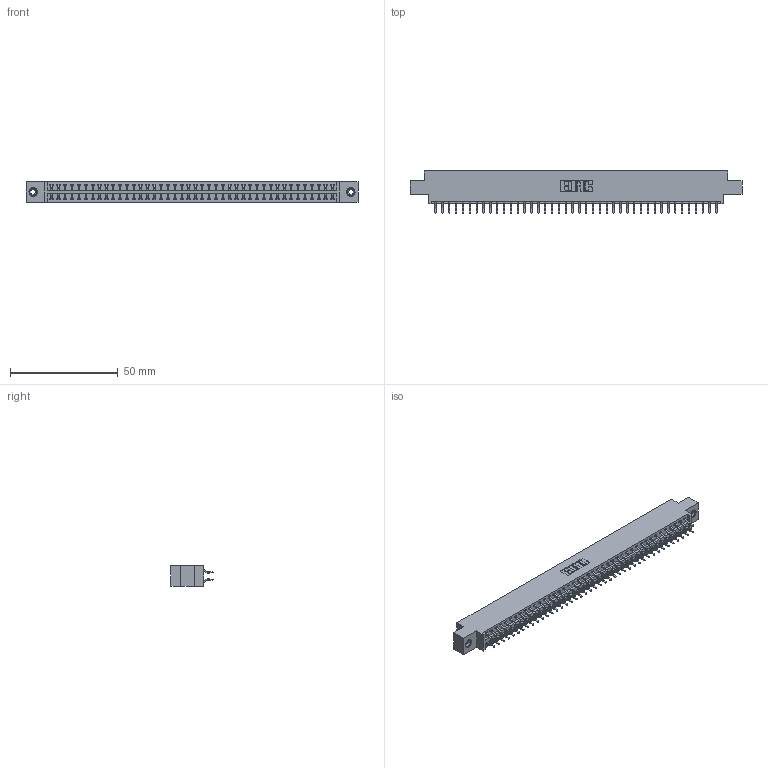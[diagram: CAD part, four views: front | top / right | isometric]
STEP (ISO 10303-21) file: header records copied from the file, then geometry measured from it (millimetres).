
FILE_DESCRIPTION (( 'STEP AP203' ), '1' );
FILE_NAME ('396-084-556-808.STEP', '2019-11-02T14:32:48', ( '' ), ( '' ), 'SwSTEP 2.0', 'SolidWorks 2016', '' );
FILE_SCHEMA (( 'CONFIG_CONTROL_DESIGN' ));
Length unit declared in the file: inch
Products named in the file (4): 345-292-001_556 Tail; 345-250-001_345-250-003-102; 396-084-556-808; 346 Part_0.170 Offset - 0.156 Dia-TI
Assembly tree (87 placements, depth 2):
  396-084-556-808
    346 Part_0.170 Offset - 0.156 Dia-TI
    345-292-001_556 Tail  x84
    345-250-001_345-250-003-102  x2
Bounding box: 153.92 x 19.57 x 9.4 mm (x, y, z)
Volume: 14845 mm3; surface area: 20527.1 mm2
Topology: 87 solids, 87 shells, 5058 faces, 15009 edges, 9886 vertices
Faces by surface type: plane 3388, cylinder 1654, cone 12, torus 4
Entity records: 28948 total; most frequent: CARTESIAN_POINT 4771, ORIENTED_EDGE 4686, DIRECTION 4269, EDGE_CURVE 2343, VECTOR 2015, LINE 2015, VERTEX_POINT 1556, AXIS2_PLACEMENT_3D 1127
